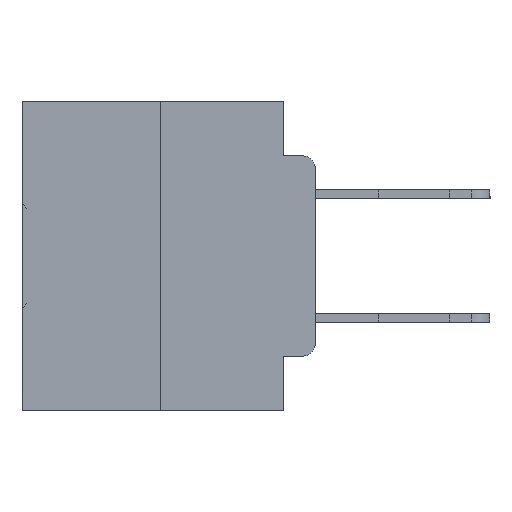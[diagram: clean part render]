
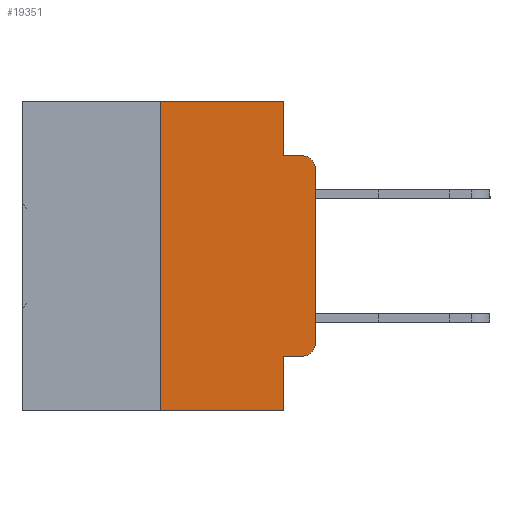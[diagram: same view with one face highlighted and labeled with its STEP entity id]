
A CAD part, left-side view. The second image highlights one B-rep face of the part: STEP entity #19351.
In plain terms, the highlighted planar face has unit normal (-1, 0, 0).
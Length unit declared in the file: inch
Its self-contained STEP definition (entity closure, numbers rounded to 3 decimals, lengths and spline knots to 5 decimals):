
#478 = VERTEX_POINT ( 'NONE', #14826 ) ;
#643 = LINE ( 'NONE', #29742, #32985 ) ;
#1621 = VECTOR ( 'NONE', #31848, 39.37008 ) ;
#2137 = LINE ( 'NONE', #29944, #14959 ) ;
#2220 = ORIENTED_EDGE ( 'NONE', *, *, #2786, .T. ) ;
#2786 = EDGE_CURVE ( 'NONE', #478, #15727, #2137, .T. ) ;
#2824 = CARTESIAN_POINT ( 'NONE',  ( 0., 0.051, -0.0885 ) ) ;
#3114 = CARTESIAN_POINT ( 'NONE',  ( 0., 0.051, -0.5 ) ) ;
#3223 = DIRECTION ( 'NONE',  ( 0., -1., 0. ) ) ;
#3325 = VERTEX_POINT ( 'NONE', #29039 ) ;
#3869 = ORIENTED_EDGE ( 'NONE', *, *, #16652, .T. ) ;
#4046 = EDGE_CURVE ( 'NONE', #5854, #18706, #27227, .T. ) ;
#4681 = DIRECTION ( 'NONE',  ( -1., 0., 0. ) ) ;
#4885 = VECTOR ( 'NONE', #16235, 39.37008 ) ;
#5002 = CARTESIAN_POINT ( 'NONE',  ( 0., 0.051, 0. ) ) ;
#5009 = DIRECTION ( 'NONE',  ( 0., 0., -1. ) ) ;
#5063 = ORIENTED_EDGE ( 'NONE', *, *, #9494, .F. ) ;
#5298 = LINE ( 'NONE', #5002, #31619 ) ;
#5854 = VERTEX_POINT ( 'NONE', #7968 ) ;
#6465 = CARTESIAN_POINT ( 'NONE',  ( 0., 0.25, 0. ) ) ;
#7031 = CARTESIAN_POINT ( 'NONE',  ( 0., 0.473, 0. ) ) ;
#7968 = CARTESIAN_POINT ( 'NONE',  ( 0., 0.02, -0.4115 ) ) ;
#8349 = CARTESIAN_POINT ( 'NONE',  ( 0., 0.051, -0.0885 ) ) ;
#8692 = ORIENTED_EDGE ( 'NONE', *, *, #27755, .F. ) ;
#9088 = ORIENTED_EDGE ( 'NONE', *, *, #9208, .F. ) ;
#9208 = EDGE_CURVE ( 'NONE', #13057, #15727, #5298, .T. ) ;
#9331 = CARTESIAN_POINT ( 'NONE',  ( 0., 0., -0.1085 ) ) ;
#9445 = EDGE_CURVE ( 'NONE', #18706, #29827, #12466, .T. ) ;
#9494 = EDGE_CURVE ( 'NONE', #28656, #3325, #10895, .T. ) ;
#9576 = DIRECTION ( 'NONE',  ( 1., 0., 0. ) ) ;
#10895 = LINE ( 'NONE', #18927, #4885 ) ;
#10897 = DIRECTION ( 'NONE',  ( 0., -1., 0. ) ) ;
#11040 = DIRECTION ( 'NONE',  ( 0., 0., 1. ) ) ;
#11405 = EDGE_LOOP ( 'NONE', ( #19034, #20614, #8692, #22223, #5063, #20234, #2220, #9088, #3869, #19067 ) ) ;
#12466 = LINE ( 'NONE', #31516, #25211 ) ;
#12616 = CARTESIAN_POINT ( 'NONE',  ( 0., 0.25, 0. ) ) ;
#12795 = DIRECTION ( 'NONE',  ( 0., 0., -1. ) ) ;
#13037 = CIRCLE ( 'NONE', #21658, 0.02 ) ;
#13057 = VERTEX_POINT ( 'NONE', #19396 ) ;
#14399 = VECTOR ( 'NONE', #5009, 39.37008 ) ;
#14826 = CARTESIAN_POINT ( 'NONE',  ( 0., 0.25, -0.5 ) ) ;
#14959 = VECTOR ( 'NONE', #3223, 39.37008 ) ;
#15727 = VERTEX_POINT ( 'NONE', #3114 ) ;
#16235 = DIRECTION ( 'NONE',  ( 0., -1., 0. ) ) ;
#16571 = CARTESIAN_POINT ( 'NONE',  ( 0., 0.02, -0.0885 ) ) ;
#16652 = EDGE_CURVE ( 'NONE', #13057, #5854, #643, .T. ) ;
#16841 = LINE ( 'NONE', #6465, #1621 ) ;
#16906 = EDGE_CURVE ( 'NONE', #29827, #23548, #13037, .T. ) ;
#16936 = AXIS2_PLACEMENT_3D ( 'NONE', #21364, #24949, #32407 ) ;
#18706 = VERTEX_POINT ( 'NONE', #19864 ) ;
#18927 = CARTESIAN_POINT ( 'NONE',  ( 0., 0.473, 0. ) ) ;
#19034 = ORIENTED_EDGE ( 'NONE', *, *, #9445, .T. ) ;
#19067 = ORIENTED_EDGE ( 'NONE', *, *, #4046, .T. ) ;
#19351 = ADVANCED_FACE ( 'NONE', ( #20060 ), #19722, .F. ) ;
#19396 = CARTESIAN_POINT ( 'NONE',  ( 0., 0.051, -0.4115 ) ) ;
#19722 = PLANE ( 'NONE',  #26440 ) ;
#19864 = CARTESIAN_POINT ( 'NONE',  ( 0., 0., -0.3915 ) ) ;
#19965 = CARTESIAN_POINT ( 'NONE',  ( 0., 0.02, -0.1085 ) ) ;
#20060 = FACE_OUTER_BOUND ( 'NONE', #11405, .T. ) ;
#20234 = ORIENTED_EDGE ( 'NONE', *, *, #27332, .F. ) ;
#20288 = CARTESIAN_POINT ( 'NONE',  ( 0., 0.051, 0. ) ) ;
#20384 = LINE ( 'NONE', #20288, #14399 ) ;
#20614 = ORIENTED_EDGE ( 'NONE', *, *, #16906, .T. ) ;
#21364 = CARTESIAN_POINT ( 'NONE',  ( 0., 0.02, -0.3915 ) ) ;
#21658 = AXIS2_PLACEMENT_3D ( 'NONE', #19965, #4681, #22533 ) ;
#22223 = ORIENTED_EDGE ( 'NONE', *, *, #24993, .F. ) ;
#22533 = DIRECTION ( 'NONE',  ( 0., 0., -1. ) ) ;
#23548 = VERTEX_POINT ( 'NONE', #16571 ) ;
#24388 = LINE ( 'NONE', #8349, #29573 ) ;
#24717 = DIRECTION ( 'NONE',  ( 0., -1., 0. ) ) ;
#24949 = DIRECTION ( 'NONE',  ( -1., 0., 0. ) ) ;
#24993 = EDGE_CURVE ( 'NONE', #3325, #25125, #20384, .T. ) ;
#25125 = VERTEX_POINT ( 'NONE', #2824 ) ;
#25211 = VECTOR ( 'NONE', #11040, 39.37008 ) ;
#26440 = AXIS2_PLACEMENT_3D ( 'NONE', #7031, #9576, #27373 ) ;
#27227 = CIRCLE ( 'NONE', #16936, 0.02 ) ;
#27332 = EDGE_CURVE ( 'NONE', #478, #28656, #16841, .T. ) ;
#27373 = DIRECTION ( 'NONE',  ( 0., 0., -1. ) ) ;
#27755 = EDGE_CURVE ( 'NONE', #25125, #23548, #24388, .T. ) ;
#28656 = VERTEX_POINT ( 'NONE', #12616 ) ;
#29039 = CARTESIAN_POINT ( 'NONE',  ( 0., 0.051, 0. ) ) ;
#29573 = VECTOR ( 'NONE', #10897, 39.37008 ) ;
#29742 = CARTESIAN_POINT ( 'NONE',  ( 0., 0.051, -0.4115 ) ) ;
#29827 = VERTEX_POINT ( 'NONE', #9331 ) ;
#29944 = CARTESIAN_POINT ( 'NONE',  ( 0., 0.473, -0.5 ) ) ;
#31516 = CARTESIAN_POINT ( 'NONE',  ( 0., 0., 0. ) ) ;
#31619 = VECTOR ( 'NONE', #12795, 39.37008 ) ;
#31848 = DIRECTION ( 'NONE',  ( 0., 0., 1. ) ) ;
#32407 = DIRECTION ( 'NONE',  ( 0., 0., -1. ) ) ;
#32985 = VECTOR ( 'NONE', #24717, 39.37008 ) ;
